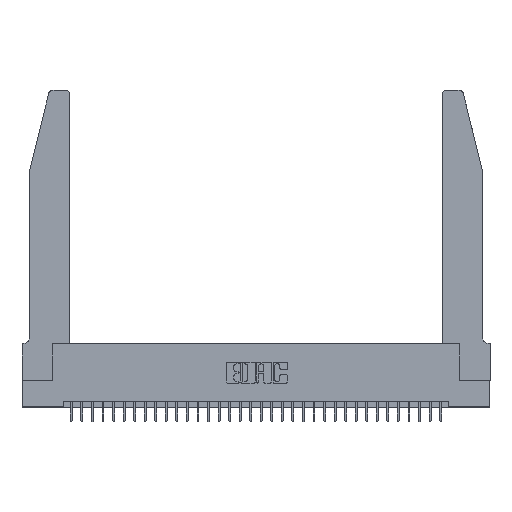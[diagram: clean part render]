
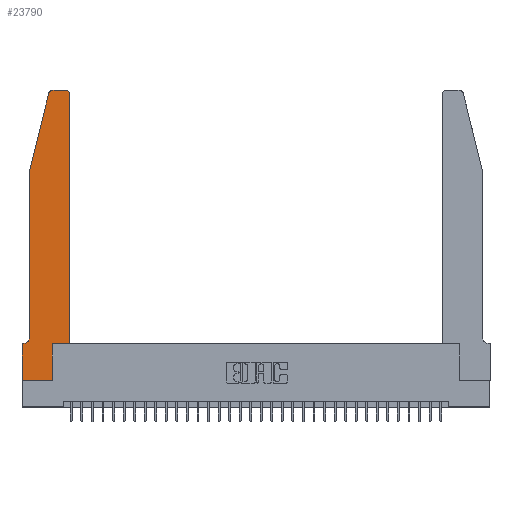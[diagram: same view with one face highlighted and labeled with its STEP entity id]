
A CAD part, top view. The second image highlights one B-rep face of the part: STEP entity #23790.
In plain terms, the highlighted planar face has unit normal (0, 0, 1).
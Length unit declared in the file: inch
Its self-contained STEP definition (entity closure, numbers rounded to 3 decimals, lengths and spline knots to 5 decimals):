
#228 = DIRECTION ( 'NONE',  ( 0., 0., -1. ) ) ;
#347 = CARTESIAN_POINT ( 'NONE',  ( 0.0755, 0.35, 0.37 ) ) ;
#516 = VERTEX_POINT ( 'NONE', #14678 ) ;
#1008 = EDGE_CURVE ( 'NONE', #23815, #28701, #23889, .T. ) ;
#1052 = AXIS2_PLACEMENT_3D ( 'NONE', #25490, #4186, #14683 ) ;
#1517 = CIRCLE ( 'NONE', #20728, 0.07 ) ;
#2348 = EDGE_CURVE ( 'NONE', #26321, #9199, #24168, .T. ) ;
#2547 = VECTOR ( 'NONE', #12180, 39.37008 ) ;
#2924 = CARTESIAN_POINT ( 'NONE',  ( 0.2865, 0.35, 0.37 ) ) ;
#3051 = VERTEX_POINT ( 'NONE', #18254 ) ;
#3240 = CARTESIAN_POINT ( 'NONE',  ( 0.0755, 2., 0.37 ) ) ;
#3267 = DIRECTION ( 'NONE',  ( 0., 1., 0. ) ) ;
#3572 = LINE ( 'NONE', #3240, #19113 ) ;
#3682 = ORIENTED_EDGE ( 'NONE', *, *, #18169, .T. ) ;
#4186 = DIRECTION ( 'NONE',  ( 0., 0., 1. ) ) ;
#4553 = CIRCLE ( 'NONE', #23759, 0.03 ) ;
#4620 = CARTESIAN_POINT ( 'NONE',  ( 0.284, 2.75, 0.37 ) ) ;
#4664 = CARTESIAN_POINT ( 'NONE',  ( 0.0055, 0.35, 0.37 ) ) ;
#5095 = CARTESIAN_POINT ( 'NONE',  ( 0.4505, 0.35, 0.37 ) ) ;
#5780 = ORIENTED_EDGE ( 'NONE', *, *, #12406, .T. ) ;
#6557 = ORIENTED_EDGE ( 'NONE', *, *, #31838, .T. ) ;
#6871 = ORIENTED_EDGE ( 'NONE', *, *, #1008, .T. ) ;
#7616 = EDGE_CURVE ( 'NONE', #33136, #516, #28460, .T. ) ;
#8820 = DIRECTION ( 'NONE',  ( -1., 0., 0. ) ) ;
#8872 = DIRECTION ( 'NONE',  ( 0., 1., 0. ) ) ;
#8898 = EDGE_CURVE ( 'NONE', #20462, #3051, #3572, .T. ) ;
#9103 = VECTOR ( 'NONE', #3267, 39.37008 ) ;
#9152 = CARTESIAN_POINT ( 'NONE',  ( 0.2605, 2.75, 0.37 ) ) ;
#9199 = VERTEX_POINT ( 'NONE', #13017 ) ;
#9383 = VECTOR ( 'NONE', #33256, 39.37008 ) ;
#9471 = CARTESIAN_POINT ( 'NONE',  ( 0.4205, 2.75, 0.37 ) ) ;
#10218 = VERTEX_POINT ( 'NONE', #21526 ) ;
#10849 = DIRECTION ( 'NONE',  ( -1., 0., 0. ) ) ;
#11015 = DIRECTION ( 'NONE',  ( 0., 0., 1. ) ) ;
#12080 = VECTOR ( 'NONE', #8872, 39.37008 ) ;
#12180 = DIRECTION ( 'NONE',  ( 1., 0., 0. ) ) ;
#12314 = LINE ( 'NONE', #20216, #20945 ) ;
#12406 = EDGE_CURVE ( 'NONE', #28701, #33136, #31026, .T. ) ;
#12842 = EDGE_CURVE ( 'NONE', #3051, #21664, #12314, .T. ) ;
#12844 = AXIS2_PLACEMENT_3D ( 'NONE', #19805, #14815, #19966 ) ;
#13017 = CARTESIAN_POINT ( 'NONE',  ( 0.4505, 2.72, 0.37 ) ) ;
#13642 = ORIENTED_EDGE ( 'NONE', *, *, #19442, .T. ) ;
#14024 = CARTESIAN_POINT ( 'NONE',  ( 0.4505, 0.35, 0.37 ) ) ;
#14143 = LINE ( 'NONE', #9152, #33252 ) ;
#14190 = DIRECTION ( 'NONE',  ( 1., 0., 0. ) ) ;
#14474 = PLANE ( 'NONE',  #12844 ) ;
#14678 = CARTESIAN_POINT ( 'NONE',  ( 0.2865, 0., 0.37 ) ) ;
#14683 = DIRECTION ( 'NONE',  ( 1., 0., 0. ) ) ;
#14815 = DIRECTION ( 'NONE',  ( 0., 0., 1. ) ) ;
#14996 = FACE_OUTER_BOUND ( 'NONE', #32834, .T. ) ;
#16172 = ORIENTED_EDGE ( 'NONE', *, *, #16179, .T. ) ;
#16179 = EDGE_CURVE ( 'NONE', #9199, #33718, #4553, .T. ) ;
#18169 = EDGE_CURVE ( 'NONE', #516, #10218, #19095, .T. ) ;
#18254 = CARTESIAN_POINT ( 'NONE',  ( 0.0755, 2., 0.37 ) ) ;
#19015 = EDGE_CURVE ( 'NONE', #10218, #26321, #28623, .T. ) ;
#19095 = LINE ( 'NONE', #2924, #9103 ) ;
#19113 = VECTOR ( 'NONE', #29850, 39.37008 ) ;
#19442 = EDGE_CURVE ( 'NONE', #21664, #23815, #1517, .T. ) ;
#19805 = CARTESIAN_POINT ( 'NONE',  ( 0., 0.35, 0.37 ) ) ;
#19966 = DIRECTION ( 'NONE',  ( 1., 0., 0. ) ) ;
#20216 = CARTESIAN_POINT ( 'NONE',  ( 0.0755, 2., 0.37 ) ) ;
#20462 = VERTEX_POINT ( 'NONE', #20802 ) ;
#20728 = AXIS2_PLACEMENT_3D ( 'NONE', #30964, #228, #21206 ) ;
#20802 = CARTESIAN_POINT ( 'NONE',  ( 0.25487, 2.72718, 0.37 ) ) ;
#20945 = VECTOR ( 'NONE', #31953, 39.37008 ) ;
#21206 = DIRECTION ( 'NONE',  ( -1., 0., 0. ) ) ;
#21526 = CARTESIAN_POINT ( 'NONE',  ( 0.2865, 0.35, 0.37 ) ) ;
#21648 = CARTESIAN_POINT ( 'NONE',  ( 0.4205, 2.72, 0.37 ) ) ;
#21664 = VERTEX_POINT ( 'NONE', #25518 ) ;
#21922 = ORIENTED_EDGE ( 'NONE', *, *, #30408, .T. ) ;
#22604 = VERTEX_POINT ( 'NONE', #4620 ) ;
#23759 = AXIS2_PLACEMENT_3D ( 'NONE', #21648, #11015, #24235 ) ;
#23790 = ADVANCED_FACE ( 'NONE', ( #14996 ), #14474, .T. ) ;
#23815 = VERTEX_POINT ( 'NONE', #4664 ) ;
#23889 = LINE ( 'NONE', #347, #31142 ) ;
#24168 = LINE ( 'NONE', #14024, #12080 ) ;
#24235 = DIRECTION ( 'NONE',  ( 1., 0., 0. ) ) ;
#25040 = CARTESIAN_POINT ( 'NONE',  ( 0., 0., 0.37 ) ) ;
#25262 = ORIENTED_EDGE ( 'NONE', *, *, #19015, .T. ) ;
#25490 = CARTESIAN_POINT ( 'NONE',  ( 0.284, 2.72, 0.37 ) ) ;
#25518 = CARTESIAN_POINT ( 'NONE',  ( 0.0755, 0.42, 0.37 ) ) ;
#25910 = CARTESIAN_POINT ( 'NONE',  ( 0., 0., 0.37 ) ) ;
#25956 = ORIENTED_EDGE ( 'NONE', *, *, #7616, .T. ) ;
#26321 = VERTEX_POINT ( 'NONE', #32354 ) ;
#26941 = ORIENTED_EDGE ( 'NONE', *, *, #8898, .T. ) ;
#28460 = LINE ( 'NONE', #25040, #2547 ) ;
#28623 = LINE ( 'NONE', #5095, #33304 ) ;
#28701 = VERTEX_POINT ( 'NONE', #32783 ) ;
#29766 = CARTESIAN_POINT ( 'NONE',  ( 0., 0., 0.37 ) ) ;
#29850 = DIRECTION ( 'NONE',  ( -0.239, -0.971, 0. ) ) ;
#30408 = EDGE_CURVE ( 'NONE', #22604, #20462, #32267, .T. ) ;
#30964 = CARTESIAN_POINT ( 'NONE',  ( 0.0055, 0.42, 0.37 ) ) ;
#31026 = LINE ( 'NONE', #25910, #9383 ) ;
#31142 = VECTOR ( 'NONE', #10849, 39.37008 ) ;
#31771 = ORIENTED_EDGE ( 'NONE', *, *, #2348, .T. ) ;
#31838 = EDGE_CURVE ( 'NONE', #33718, #22604, #14143, .T. ) ;
#31953 = DIRECTION ( 'NONE',  ( 0., -1., 0. ) ) ;
#32267 = CIRCLE ( 'NONE', #1052, 0.03 ) ;
#32354 = CARTESIAN_POINT ( 'NONE',  ( 0.4505, 0.35, 0.37 ) ) ;
#32783 = CARTESIAN_POINT ( 'NONE',  ( 0., 0.35, 0.37 ) ) ;
#32834 = EDGE_LOOP ( 'NONE', ( #6557, #21922, #26941, #33020, #13642, #6871, #5780, #25956, #3682, #25262, #31771, #16172 ) ) ;
#33020 = ORIENTED_EDGE ( 'NONE', *, *, #12842, .T. ) ;
#33136 = VERTEX_POINT ( 'NONE', #29766 ) ;
#33252 = VECTOR ( 'NONE', #8820, 39.37008 ) ;
#33256 = DIRECTION ( 'NONE',  ( 0., -1., 0. ) ) ;
#33304 = VECTOR ( 'NONE', #14190, 39.37008 ) ;
#33718 = VERTEX_POINT ( 'NONE', #9471 ) ;
